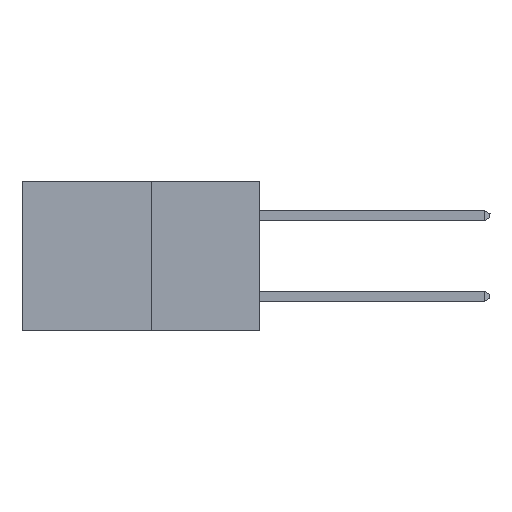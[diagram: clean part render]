
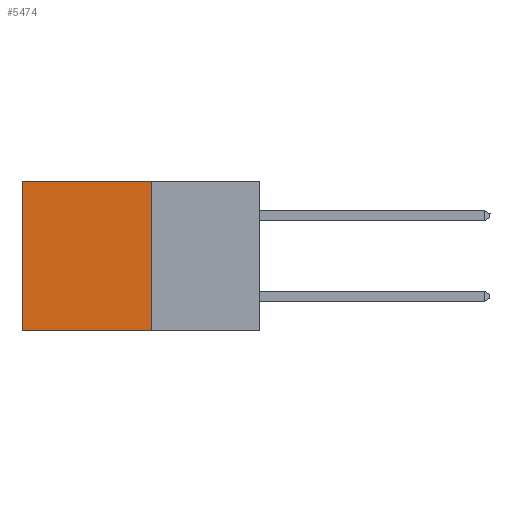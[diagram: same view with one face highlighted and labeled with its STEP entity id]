
A CAD part, left-side view. The second image highlights one B-rep face of the part: STEP entity #5474.
In plain terms, the highlighted planar face has unit normal (-1, 0, 0).
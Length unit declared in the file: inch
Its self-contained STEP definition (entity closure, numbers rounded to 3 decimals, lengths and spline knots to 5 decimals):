
#16 = EDGE_CURVE ( 'NONE', #2566, #4791, #6231, .T. ) ;
#92 = AXIS2_PLACEMENT_3D ( 'NONE', #5992, #5990, #3197 ) ;
#401 = CARTESIAN_POINT ( 'NONE',  ( 0.277, 0.27, -0.37 ) ) ;
#502 = ORIENTED_EDGE ( 'NONE', *, *, #3210, .T. ) ;
#660 = CARTESIAN_POINT ( 'NONE',  ( 0.277, 0.27, -0.37 ) ) ;
#1573 = VERTEX_POINT ( 'NONE', #6914 ) ;
#1577 = FACE_OUTER_BOUND ( 'NONE', #6182, .T. ) ;
#2203 = VECTOR ( 'NONE', #3538, 39.37008 ) ;
#2436 = ORIENTED_EDGE ( 'NONE', *, *, #3840, .T. ) ;
#2566 = VERTEX_POINT ( 'NONE', #6719 ) ;
#2649 = VERTEX_POINT ( 'NONE', #8473 ) ;
#3102 = VECTOR ( 'NONE', #3370, 39.37008 ) ;
#3187 = ORIENTED_EDGE ( 'NONE', *, *, #16, .F. ) ;
#3197 = DIRECTION ( 'NONE',  ( 0., 0., -1. ) ) ;
#3210 = EDGE_CURVE ( 'NONE', #2649, #1573, #4977, .T. ) ;
#3370 = DIRECTION ( 'NONE',  ( 0., 1., 0. ) ) ;
#3538 = DIRECTION ( 'NONE',  ( 0., 1., 0. ) ) ;
#3785 = DIRECTION ( 'NONE',  ( 0., 0., -1. ) ) ;
#3840 = EDGE_CURVE ( 'NONE', #2566, #2649, #4085, .T. ) ;
#3965 = CARTESIAN_POINT ( 'NONE',  ( 0.277, 0.59, -0.37 ) ) ;
#4085 = LINE ( 'NONE', #6145, #2203 ) ;
#4347 = VECTOR ( 'NONE', #4427, 39.37008 ) ;
#4427 = DIRECTION ( 'NONE',  ( 0., 0., -1. ) ) ;
#4572 = PLANE ( 'NONE',  #92 ) ;
#4699 = CARTESIAN_POINT ( 'NONE',  ( 0.277, 0.27, -0.37 ) ) ;
#4791 = VERTEX_POINT ( 'NONE', #660 ) ;
#4977 = LINE ( 'NONE', #3965, #8351 ) ;
#5385 = ORIENTED_EDGE ( 'NONE', *, *, #6404, .F. ) ;
#5474 = ADVANCED_FACE ( 'NONE', ( #1577 ), #4572, .F. ) ;
#5990 = DIRECTION ( 'NONE',  ( 1., 0., 0. ) ) ;
#5992 = CARTESIAN_POINT ( 'NONE',  ( 0.277, 0.27, -0.37 ) ) ;
#6145 = CARTESIAN_POINT ( 'NONE',  ( 0.277, 0.27, 0. ) ) ;
#6182 = EDGE_LOOP ( 'NONE', ( #502, #5385, #3187, #2436 ) ) ;
#6231 = LINE ( 'NONE', #4699, #4347 ) ;
#6404 = EDGE_CURVE ( 'NONE', #4791, #1573, #6903, .T. ) ;
#6719 = CARTESIAN_POINT ( 'NONE',  ( 0.277, 0.27, 0. ) ) ;
#6903 = LINE ( 'NONE', #401, #3102 ) ;
#6914 = CARTESIAN_POINT ( 'NONE',  ( 0.277, 0.59, -0.37 ) ) ;
#8351 = VECTOR ( 'NONE', #3785, 39.37008 ) ;
#8473 = CARTESIAN_POINT ( 'NONE',  ( 0.277, 0.59, 0. ) ) ;
